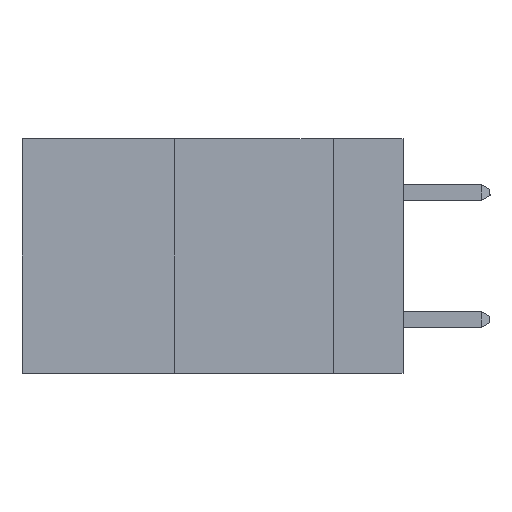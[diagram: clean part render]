
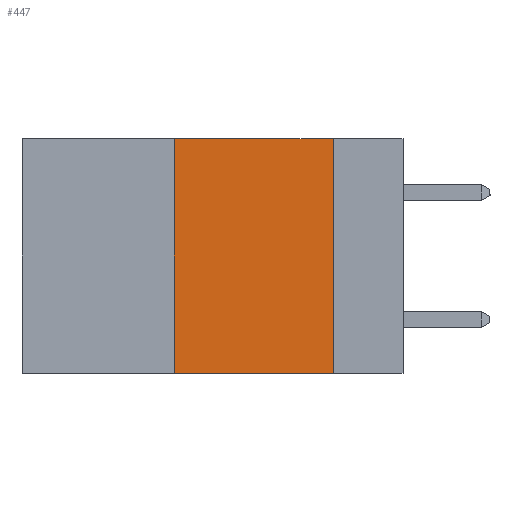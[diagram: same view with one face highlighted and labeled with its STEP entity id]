
A CAD part, left-side view. The second image highlights one B-rep face of the part: STEP entity #447.
In plain terms, the highlighted planar face has unit normal (-1, 0, 0).
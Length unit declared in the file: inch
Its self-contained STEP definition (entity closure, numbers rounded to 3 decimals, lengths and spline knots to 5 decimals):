
#135 = VERTEX_POINT ( 'NONE', #9220 ) ;
#447 = ADVANCED_FACE ( 'NONE', ( #9758 ), #5614, .F. ) ;
#611 = VERTEX_POINT ( 'NONE', #7855 ) ;
#663 = CARTESIAN_POINT ( 'NONE',  ( 0., 0.6, 0. ) ) ;
#974 = DIRECTION ( 'NONE',  ( 0., -1., 0. ) ) ;
#1323 = VECTOR ( 'NONE', #8582, 39.37008 ) ;
#1859 = LINE ( 'NONE', #4419, #1323 ) ;
#2125 = EDGE_LOOP ( 'NONE', ( #3978, #9410, #9797, #7694 ) ) ;
#3130 = CARTESIAN_POINT ( 'NONE',  ( 0., 0.36, -0.37 ) ) ;
#3310 = CARTESIAN_POINT ( 'NONE',  ( 0., 0.36, 0. ) ) ;
#3322 = EDGE_CURVE ( 'NONE', #611, #9586, #6495, .T. ) ;
#3464 = CARTESIAN_POINT ( 'NONE',  ( 0., 0.6, -0.37 ) ) ;
#3918 = DIRECTION ( 'NONE',  ( 0., -1., 0. ) ) ;
#3965 = DIRECTION ( 'NONE',  ( 0., 0., -1. ) ) ;
#3978 = ORIENTED_EDGE ( 'NONE', *, *, #5125, .F. ) ;
#4419 = CARTESIAN_POINT ( 'NONE',  ( 0., 0.11, 0. ) ) ;
#5125 = EDGE_CURVE ( 'NONE', #9586, #135, #1859, .T. ) ;
#5496 = VECTOR ( 'NONE', #3918, 39.37008 ) ;
#5564 = VECTOR ( 'NONE', #7358, 39.37008 ) ;
#5614 = PLANE ( 'NONE',  #7076 ) ;
#6245 = VECTOR ( 'NONE', #974, 39.37008 ) ;
#6495 = LINE ( 'NONE', #10476, #5496 ) ;
#6801 = LINE ( 'NONE', #3464, #6245 ) ;
#7076 = AXIS2_PLACEMENT_3D ( 'NONE', #663, #8137, #3965 ) ;
#7358 = DIRECTION ( 'NONE',  ( 0., 0., 1. ) ) ;
#7553 = CARTESIAN_POINT ( 'NONE',  ( 0., 0.11, 0. ) ) ;
#7651 = EDGE_CURVE ( 'NONE', #10467, #135, #6801, .T. ) ;
#7694 = ORIENTED_EDGE ( 'NONE', *, *, #7651, .T. ) ;
#7855 = CARTESIAN_POINT ( 'NONE',  ( 0., 0.36, 0. ) ) ;
#8137 = DIRECTION ( 'NONE',  ( 1., 0., 0. ) ) ;
#8349 = LINE ( 'NONE', #3310, #5564 ) ;
#8582 = DIRECTION ( 'NONE',  ( 0., 0., -1. ) ) ;
#8654 = EDGE_CURVE ( 'NONE', #10467, #611, #8349, .T. ) ;
#9220 = CARTESIAN_POINT ( 'NONE',  ( 0., 0.11, -0.37 ) ) ;
#9410 = ORIENTED_EDGE ( 'NONE', *, *, #3322, .F. ) ;
#9586 = VERTEX_POINT ( 'NONE', #7553 ) ;
#9758 = FACE_OUTER_BOUND ( 'NONE', #2125, .T. ) ;
#9797 = ORIENTED_EDGE ( 'NONE', *, *, #8654, .F. ) ;
#10467 = VERTEX_POINT ( 'NONE', #3130 ) ;
#10476 = CARTESIAN_POINT ( 'NONE',  ( 0., 0.6, 0. ) ) ;
